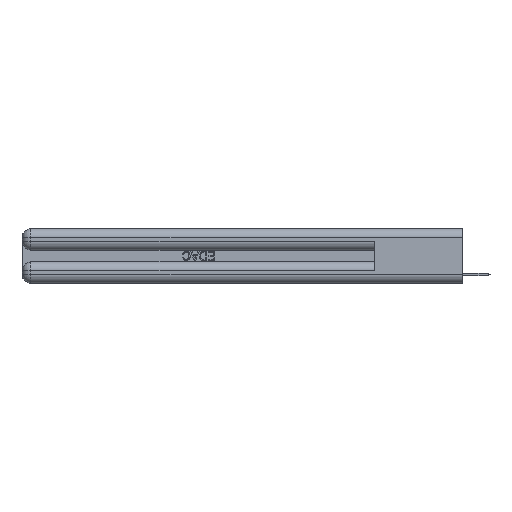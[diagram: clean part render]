
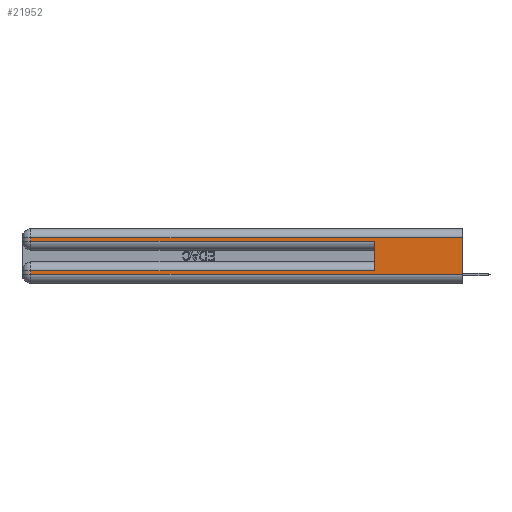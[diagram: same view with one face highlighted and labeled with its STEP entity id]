
A CAD part, left-side view. The second image highlights one B-rep face of the part: STEP entity #21952.
In plain terms, the highlighted planar face has unit normal (-1, 0, 0).
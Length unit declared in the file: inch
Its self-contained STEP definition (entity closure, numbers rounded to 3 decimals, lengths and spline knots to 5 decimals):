
#27 = VERTEX_POINT ( 'NONE', #17483 ) ;
#812 = LINE ( 'NONE', #18666, #27515 ) ;
#1094 = LINE ( 'NONE', #9676, #6691 ) ;
#1174 = ORIENTED_EDGE ( 'NONE', *, *, #26109, .T. ) ;
#1304 = VERTEX_POINT ( 'NONE', #27273 ) ;
#1764 = DIRECTION ( 'NONE',  ( 1., 0., 0. ) ) ;
#1829 = DIRECTION ( 'NONE',  ( 0., -1., 0. ) ) ;
#2365 = CARTESIAN_POINT ( 'NONE',  ( 0., 0., 0.37 ) ) ;
#2511 = DIRECTION ( 'NONE',  ( 0., 0., -1. ) ) ;
#3161 = EDGE_CURVE ( 'NONE', #15719, #7396, #27235, .T. ) ;
#3372 = VERTEX_POINT ( 'NONE', #8276 ) ;
#3711 = VECTOR ( 'NONE', #8006, 39.37008 ) ;
#3825 = AXIS2_PLACEMENT_3D ( 'NONE', #28803, #1764, #17115 ) ;
#3843 = CARTESIAN_POINT ( 'NONE',  ( 0., 0., 0.06 ) ) ;
#5468 = CARTESIAN_POINT ( 'NONE',  ( 0., 0., 0.31 ) ) ;
#5757 = VECTOR ( 'NONE', #14074, 39.37008 ) ;
#6656 = VECTOR ( 'NONE', #13001, 39.37008 ) ;
#6684 = CARTESIAN_POINT ( 'NONE',  ( 0., 2.94, 0.37 ) ) ;
#6691 = VECTOR ( 'NONE', #25851, 39.37008 ) ;
#6916 = EDGE_CURVE ( 'NONE', #15719, #27130, #812, .T. ) ;
#7396 = VERTEX_POINT ( 'NONE', #3843 ) ;
#7567 = ORIENTED_EDGE ( 'NONE', *, *, #17637, .T. ) ;
#7652 = CARTESIAN_POINT ( 'NONE',  ( 0., 0.6, 0.085 ) ) ;
#7963 = VERTEX_POINT ( 'NONE', #11546 ) ;
#8006 = DIRECTION ( 'NONE',  ( 0., 1., 0. ) ) ;
#8276 = CARTESIAN_POINT ( 'NONE',  ( 0., 2.94, 0.285 ) ) ;
#8316 = CARTESIAN_POINT ( 'NONE',  ( 0., 0., 0.285 ) ) ;
#9676 = CARTESIAN_POINT ( 'NONE',  ( 0., 0.6, 0.145 ) ) ;
#9723 = ORIENTED_EDGE ( 'NONE', *, *, #26977, .F. ) ;
#9929 = LINE ( 'NONE', #25386, #5757 ) ;
#10583 = EDGE_CURVE ( 'NONE', #27130, #3372, #19913, .T. ) ;
#11546 = CARTESIAN_POINT ( 'NONE',  ( 0., 2.94, 0.06 ) ) ;
#13001 = DIRECTION ( 'NONE',  ( 0., -1., 0. ) ) ;
#14074 = DIRECTION ( 'NONE',  ( 0., 0., -1. ) ) ;
#15070 = FACE_OUTER_BOUND ( 'NONE', #20523, .T. ) ;
#15644 = DIRECTION ( 'NONE',  ( 0., 0., -1. ) ) ;
#15719 = VERTEX_POINT ( 'NONE', #5468 ) ;
#16482 = VERTEX_POINT ( 'NONE', #7652 ) ;
#17115 = DIRECTION ( 'NONE',  ( 0., 0., -1. ) ) ;
#17208 = ORIENTED_EDGE ( 'NONE', *, *, #10583, .T. ) ;
#17483 = CARTESIAN_POINT ( 'NONE',  ( 0., 2.94, 0.085 ) ) ;
#17637 = EDGE_CURVE ( 'NONE', #16482, #27, #28531, .T. ) ;
#18666 = CARTESIAN_POINT ( 'NONE',  ( 0., 0., 0.31 ) ) ;
#19445 = ORIENTED_EDGE ( 'NONE', *, *, #28750, .T. ) ;
#19540 = CARTESIAN_POINT ( 'NONE',  ( 0., 0., 0.06 ) ) ;
#19741 = ORIENTED_EDGE ( 'NONE', *, *, #3161, .F. ) ;
#19913 = LINE ( 'NONE', #6684, #27111 ) ;
#20523 = EDGE_LOOP ( 'NONE', ( #19741, #26057, #17208, #1174, #9723, #7567, #19445, #28527 ) ) ;
#21952 = ADVANCED_FACE ( 'NONE', ( #15070 ), #22116, .F. ) ;
#22116 = PLANE ( 'NONE',  #3825 ) ;
#23177 = CARTESIAN_POINT ( 'NONE',  ( 0., 2.94, 0.31 ) ) ;
#23361 = DIRECTION ( 'NONE',  ( 0., 1., 0. ) ) ;
#25013 = VECTOR ( 'NONE', #1829, 39.37008 ) ;
#25386 = CARTESIAN_POINT ( 'NONE',  ( 0., 2.94, 0.37 ) ) ;
#25851 = DIRECTION ( 'NONE',  ( 0., 0., 1. ) ) ;
#26057 = ORIENTED_EDGE ( 'NONE', *, *, #6916, .T. ) ;
#26109 = EDGE_CURVE ( 'NONE', #3372, #1304, #28417, .T. ) ;
#26548 = LINE ( 'NONE', #19540, #25013 ) ;
#26659 = VECTOR ( 'NONE', #2511, 39.37008 ) ;
#26977 = EDGE_CURVE ( 'NONE', #16482, #1304, #1094, .T. ) ;
#27111 = VECTOR ( 'NONE', #15644, 39.37008 ) ;
#27130 = VERTEX_POINT ( 'NONE', #23177 ) ;
#27235 = LINE ( 'NONE', #2365, #26659 ) ;
#27273 = CARTESIAN_POINT ( 'NONE',  ( 0., 0.6, 0.285 ) ) ;
#27515 = VECTOR ( 'NONE', #23361, 39.37008 ) ;
#27696 = EDGE_CURVE ( 'NONE', #7963, #7396, #26548, .T. ) ;
#27976 = CARTESIAN_POINT ( 'NONE',  ( 0., 0., 0.085 ) ) ;
#28417 = LINE ( 'NONE', #8316, #6656 ) ;
#28527 = ORIENTED_EDGE ( 'NONE', *, *, #27696, .T. ) ;
#28531 = LINE ( 'NONE', #27976, #3711 ) ;
#28750 = EDGE_CURVE ( 'NONE', #27, #7963, #9929, .T. ) ;
#28803 = CARTESIAN_POINT ( 'NONE',  ( 0., 0., 0.37 ) ) ;
